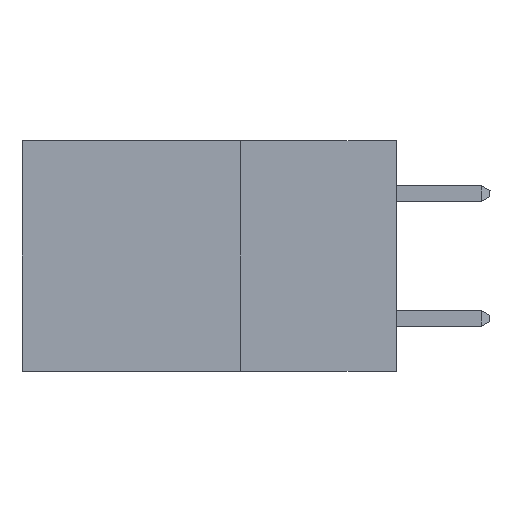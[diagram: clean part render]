
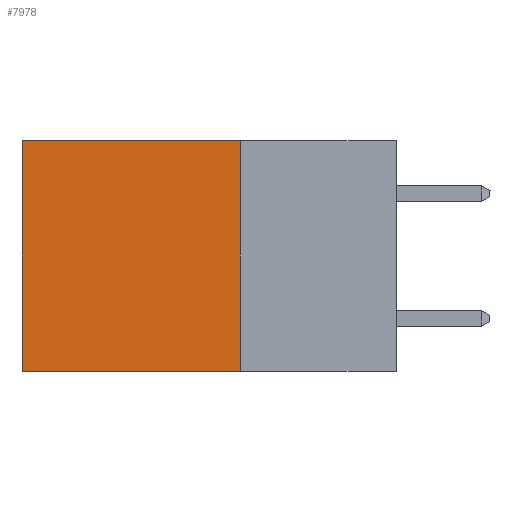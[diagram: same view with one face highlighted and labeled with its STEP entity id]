
A CAD part, left-side view. The second image highlights one B-rep face of the part: STEP entity #7978.
In plain terms, the highlighted planar face has unit normal (-1, 0, 0).
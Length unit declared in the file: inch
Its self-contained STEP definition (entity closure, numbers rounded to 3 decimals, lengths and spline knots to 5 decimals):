
#217 = EDGE_CURVE ( 'NONE', #23195, #25843, #31081, .T. ) ;
#1787 = LINE ( 'NONE', #28870, #28270 ) ;
#2680 = CARTESIAN_POINT ( 'NONE',  ( 0.298, 0.25, -0.37 ) ) ;
#4689 = CARTESIAN_POINT ( 'NONE',  ( 0.298, 0.25, 0. ) ) ;
#5449 = AXIS2_PLACEMENT_3D ( 'NONE', #13159, #8010, #26018 ) ;
#6025 = ORIENTED_EDGE ( 'NONE', *, *, #28627, .T. ) ;
#6278 = EDGE_CURVE ( 'NONE', #17290, #25843, #30056, .T. ) ;
#7259 = DIRECTION ( 'NONE',  ( 0., 0., -1. ) ) ;
#7758 = VECTOR ( 'NONE', #7259, 39.37008 ) ;
#7978 = ADVANCED_FACE ( 'NONE', ( #26781 ), #15755, .F. ) ;
#8010 = DIRECTION ( 'NONE',  ( 1., 0., 0. ) ) ;
#10459 = VECTOR ( 'NONE', #25829, 39.37008 ) ;
#10710 = VECTOR ( 'NONE', #16865, 39.37008 ) ;
#11924 = ORIENTED_EDGE ( 'NONE', *, *, #217, .T. ) ;
#12262 = ORIENTED_EDGE ( 'NONE', *, *, #6278, .F. ) ;
#13159 = CARTESIAN_POINT ( 'NONE',  ( 0.298, 0.25, 0. ) ) ;
#13629 = ORIENTED_EDGE ( 'NONE', *, *, #25564, .F. ) ;
#14708 = LINE ( 'NONE', #4689, #7758 ) ;
#15755 = PLANE ( 'NONE',  #5449 ) ;
#16107 = CARTESIAN_POINT ( 'NONE',  ( 0.298, 0.6, -0.37 ) ) ;
#16865 = DIRECTION ( 'NONE',  ( 0., 0., -1. ) ) ;
#17290 = VERTEX_POINT ( 'NONE', #2680 ) ;
#17811 = VERTEX_POINT ( 'NONE', #27654 ) ;
#21956 = CARTESIAN_POINT ( 'NONE',  ( 0.298, 0.6, 0. ) ) ;
#23195 = VERTEX_POINT ( 'NONE', #32680 ) ;
#23287 = CARTESIAN_POINT ( 'NONE',  ( 0.298, 0.25, -0.37 ) ) ;
#25564 = EDGE_CURVE ( 'NONE', #17811, #17290, #14708, .T. ) ;
#25829 = DIRECTION ( 'NONE',  ( 0., 1., 0. ) ) ;
#25843 = VERTEX_POINT ( 'NONE', #16107 ) ;
#26018 = DIRECTION ( 'NONE',  ( 0., 0., -1. ) ) ;
#26781 = FACE_OUTER_BOUND ( 'NONE', #28114, .T. ) ;
#27654 = CARTESIAN_POINT ( 'NONE',  ( 0.298, 0.25, 0. ) ) ;
#28114 = EDGE_LOOP ( 'NONE', ( #11924, #12262, #13629, #6025 ) ) ;
#28270 = VECTOR ( 'NONE', #31439, 39.37008 ) ;
#28627 = EDGE_CURVE ( 'NONE', #17811, #23195, #1787, .T. ) ;
#28870 = CARTESIAN_POINT ( 'NONE',  ( 0.298, 0.25, 0. ) ) ;
#30056 = LINE ( 'NONE', #23287, #10459 ) ;
#31081 = LINE ( 'NONE', #21956, #10710 ) ;
#31439 = DIRECTION ( 'NONE',  ( 0., 1., 0. ) ) ;
#32680 = CARTESIAN_POINT ( 'NONE',  ( 0.298, 0.6, 0. ) ) ;
